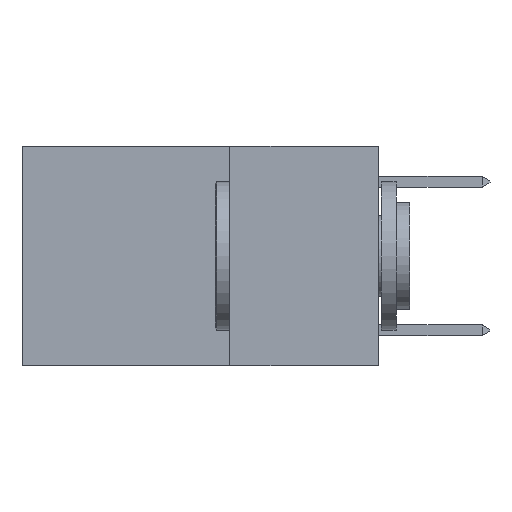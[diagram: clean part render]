
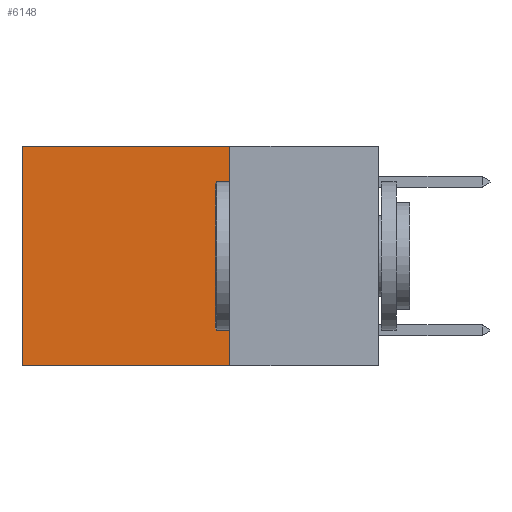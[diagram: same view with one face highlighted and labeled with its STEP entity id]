
A CAD part, left-side view. The second image highlights one B-rep face of the part: STEP entity #6148.
In plain terms, the highlighted planar face has unit normal (-1, 0, 0).
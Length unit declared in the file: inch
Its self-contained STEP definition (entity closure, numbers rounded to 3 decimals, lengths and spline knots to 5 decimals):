
#374 = ORIENTED_EDGE ( 'NONE', *, *, #1899, .T. ) ;
#551 = DIRECTION ( 'NONE',  ( 0., 0., -1. ) ) ;
#715 = EDGE_CURVE ( 'NONE', #3867, #7333, #4852, .T. ) ;
#1201 = DIRECTION ( 'NONE',  ( 0., 0., -1. ) ) ;
#1295 = VECTOR ( 'NONE', #551, 39.37008 ) ;
#1356 = EDGE_LOOP ( 'NONE', ( #8149, #4733, #5517, #374 ) ) ;
#1418 = LINE ( 'NONE', #6504, #3481 ) ;
#1766 = LINE ( 'NONE', #5655, #1295 ) ;
#1899 = EDGE_CURVE ( 'NONE', #4165, #3867, #3238, .T. ) ;
#1968 = CARTESIAN_POINT ( 'NONE',  ( 0.2625, 0.6, 0. ) ) ;
#2438 = CARTESIAN_POINT ( 'NONE',  ( 0.2625, 0.6, 0. ) ) ;
#2556 = PLANE ( 'NONE',  #3507 ) ;
#2639 = EDGE_CURVE ( 'NONE', #4798, #7333, #1418, .T. ) ;
#3238 = LINE ( 'NONE', #5523, #6340 ) ;
#3481 = VECTOR ( 'NONE', #9446, 39.37008 ) ;
#3507 = AXIS2_PLACEMENT_3D ( 'NONE', #6351, #9151, #7683 ) ;
#3867 = VERTEX_POINT ( 'NONE', #2438 ) ;
#3877 = EDGE_CURVE ( 'NONE', #4165, #4798, #1766, .T. ) ;
#4165 = VERTEX_POINT ( 'NONE', #4415 ) ;
#4415 = CARTESIAN_POINT ( 'NONE',  ( 0.2625, 0.25, 0. ) ) ;
#4733 = ORIENTED_EDGE ( 'NONE', *, *, #2639, .F. ) ;
#4798 = VERTEX_POINT ( 'NONE', #6856 ) ;
#4852 = LINE ( 'NONE', #1968, #7691 ) ;
#5517 = ORIENTED_EDGE ( 'NONE', *, *, #3877, .F. ) ;
#5523 = CARTESIAN_POINT ( 'NONE',  ( 0.2625, 0.25, 0. ) ) ;
#5588 = FACE_OUTER_BOUND ( 'NONE', #1356, .T. ) ;
#5655 = CARTESIAN_POINT ( 'NONE',  ( 0.2625, 0.25, 0. ) ) ;
#6148 = ADVANCED_FACE ( 'NONE', ( #5588 ), #2556, .F. ) ;
#6340 = VECTOR ( 'NONE', #9081, 39.37008 ) ;
#6351 = CARTESIAN_POINT ( 'NONE',  ( 0.2625, 0.25, 0. ) ) ;
#6504 = CARTESIAN_POINT ( 'NONE',  ( 0.2625, 0.25, -0.37 ) ) ;
#6856 = CARTESIAN_POINT ( 'NONE',  ( 0.2625, 0.25, -0.37 ) ) ;
#7333 = VERTEX_POINT ( 'NONE', #7454 ) ;
#7454 = CARTESIAN_POINT ( 'NONE',  ( 0.2625, 0.6, -0.37 ) ) ;
#7683 = DIRECTION ( 'NONE',  ( 0., 0., -1. ) ) ;
#7691 = VECTOR ( 'NONE', #1201, 39.37008 ) ;
#8149 = ORIENTED_EDGE ( 'NONE', *, *, #715, .T. ) ;
#9081 = DIRECTION ( 'NONE',  ( 0., 1., 0. ) ) ;
#9151 = DIRECTION ( 'NONE',  ( 1., 0., 0. ) ) ;
#9446 = DIRECTION ( 'NONE',  ( 0., 1., 0. ) ) ;
